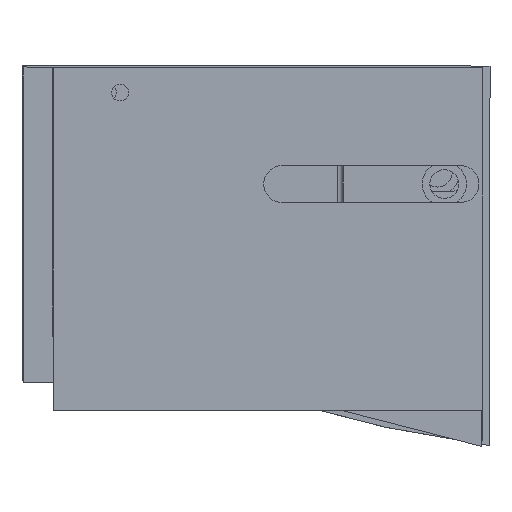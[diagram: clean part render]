
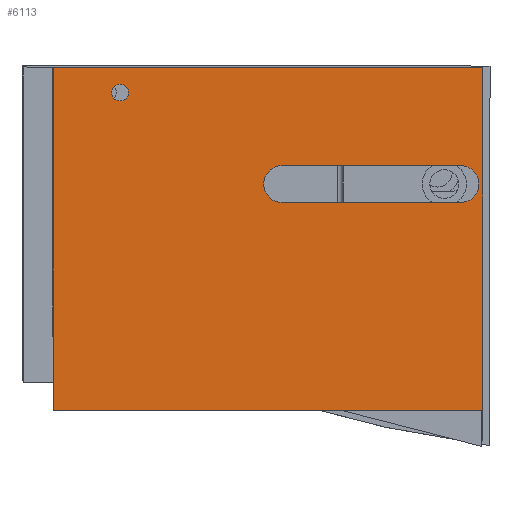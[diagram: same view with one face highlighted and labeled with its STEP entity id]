
A CAD part, left-side view. The second image highlights one B-rep face of the part: STEP entity #6113.
In plain terms, the highlighted face is planar.
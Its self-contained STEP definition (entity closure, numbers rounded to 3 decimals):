
#293=FACE_BOUND('',#1094,.T.);
#294=FACE_BOUND('',#1095,.T.);
#447=CIRCLE('',#6638,3.315);
#448=CIRCLE('',#6639,3.315);
#449=CIRCLE('',#6640,1.5);
#739=FACE_OUTER_BOUND('',#1093,.T.);
#1093=EDGE_LOOP('',(#4899,#4900,#4901,#4902));
#1094=EDGE_LOOP('',(#4903,#4904,#4905,#4906));
#1095=EDGE_LOOP('',(#4907));
#1585=LINE('',#10325,#2199);
#1596=LINE('',#10362,#2210);
#1604=LINE('',#10392,#2218);
#1616=LINE('',#10434,#2230);
#1617=LINE('',#10437,#2231);
#1618=LINE('',#10441,#2232);
#2199=VECTOR('',#7715,10.);
#2210=VECTOR('',#7744,10.);
#2218=VECTOR('',#7768,10.);
#2230=VECTOR('',#7800,10.);
#2231=VECTOR('',#7801,10.);
#2232=VECTOR('',#7804,10.);
#2806=VERTEX_POINT('',#10321);
#2808=VERTEX_POINT('',#10324);
#2825=VERTEX_POINT('',#10360);
#2833=VERTEX_POINT('',#10390);
#2854=VERTEX_POINT('',#10435);
#2855=VERTEX_POINT('',#10436);
#2856=VERTEX_POINT('',#10438);
#2857=VERTEX_POINT('',#10440);
#2858=VERTEX_POINT('',#10443);
#3536=EDGE_CURVE('',#2806,#2808,#1585,.T.);
#3555=EDGE_CURVE('',#2806,#2825,#1596,.T.);
#3568=EDGE_CURVE('',#2833,#2825,#1604,.T.);
#3589=EDGE_CURVE('',#2808,#2833,#1616,.T.);
#3590=EDGE_CURVE('',#2854,#2855,#1617,.T.);
#3591=EDGE_CURVE('',#2855,#2856,#447,.T.);
#3592=EDGE_CURVE('',#2856,#2857,#1618,.F.);
#3593=EDGE_CURVE('',#2857,#2854,#448,.T.);
#3594=EDGE_CURVE('',#2858,#2858,#449,.T.);
#4899=ORIENTED_EDGE('',*,*,#3536,.F.);
#4900=ORIENTED_EDGE('',*,*,#3555,.T.);
#4901=ORIENTED_EDGE('',*,*,#3568,.F.);
#4902=ORIENTED_EDGE('',*,*,#3589,.F.);
#4903=ORIENTED_EDGE('',*,*,#3590,.T.);
#4904=ORIENTED_EDGE('',*,*,#3591,.T.);
#4905=ORIENTED_EDGE('',*,*,#3592,.T.);
#4906=ORIENTED_EDGE('',*,*,#3593,.T.);
#4907=ORIENTED_EDGE('',*,*,#3594,.F.);
#5863=PLANE('',#6637);
#6113=ADVANCED_FACE('',(#739,#293,#294),#5863,.F.);
#6637=AXIS2_PLACEMENT_3D('',#10433,#7798,#7799);
#6638=AXIS2_PLACEMENT_3D('',#10439,#7802,#7803);
#6639=AXIS2_PLACEMENT_3D('',#10442,#7805,#7806);
#6640=AXIS2_PLACEMENT_3D('',#10444,#7807,#7808);
#7715=DIRECTION('',(0.,-1.,0.));
#7744=DIRECTION('',(0.,0.,1.));
#7768=DIRECTION('',(0.,1.,-0.001));
#7798=DIRECTION('center_axis',(-1.,0.,0.));
#7799=DIRECTION('ref_axis',(0.,1.,0.));
#7800=DIRECTION('',(0.,0.,1.));
#7801=DIRECTION('',(0.,1.,0.));
#7802=DIRECTION('center_axis',(-1.,0.,0.));
#7803=DIRECTION('ref_axis',(0.,0.,-1.));
#7804=DIRECTION('',(0.,1.,0.));
#7805=DIRECTION('center_axis',(-1.,0.,0.));
#7806=DIRECTION('ref_axis',(0.,0.,1.));
#7807=DIRECTION('center_axis',(1.,0.,0.));
#7808=DIRECTION('ref_axis',(0.,-1.,0.));
#10321=CARTESIAN_POINT('',(15.24,-75.158,-101.05));
#10324=CARTESIAN_POINT('',(15.24,-152.158,-101.05));
#10325=CARTESIAN_POINT('',(15.24,-142.862,-101.05));
#10360=CARTESIAN_POINT('',(15.24,-75.158,-39.59));
#10362=CARTESIAN_POINT('',(15.24,-75.158,-58.05));
#10390=CARTESIAN_POINT('',(15.24,-152.158,-39.531));
#10392=CARTESIAN_POINT('',(15.24,-96.377,-39.574));
#10433=CARTESIAN_POINT('Origin',(15.24,-140.158,-44.05));
#10434=CARTESIAN_POINT('',(15.24,-152.158,-48.555));
#10435=CARTESIAN_POINT('',(15.24,-111.11,-57.134));
#10436=CARTESIAN_POINT('',(15.24,-79.112,-57.134));
#10437=CARTESIAN_POINT('',(15.24,-99.632,-57.134));
#10438=CARTESIAN_POINT('',(15.24,-79.112,-63.764));
#10439=CARTESIAN_POINT('Origin',(15.24,-79.112,-60.449));
#10440=CARTESIAN_POINT('',(15.24,-111.11,-63.764));
#10441=CARTESIAN_POINT('',(15.24,-110.131,-63.764));
#10442=CARTESIAN_POINT('Origin',(15.24,-111.091,-60.449));
#10443=CARTESIAN_POINT('',(15.24,-138.658,-44.05));
#10444=CARTESIAN_POINT('Origin',(15.24,-140.158,-44.05));
